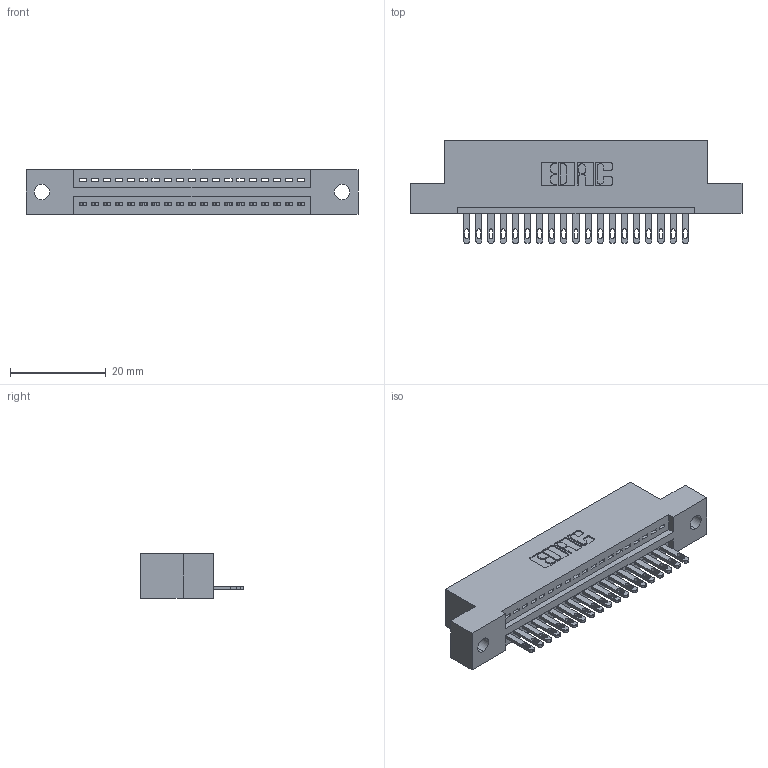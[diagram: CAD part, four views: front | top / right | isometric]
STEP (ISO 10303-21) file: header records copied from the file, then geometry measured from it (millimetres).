
FILE_DESCRIPTION (( 'STEP AP203' ), '1' );
FILE_NAME ('895-019-500-102.STEP', '2020-09-25T06:59:37', ( '' ), ( '' ), 'SwSTEP 2.0', 'SolidWorks 2020', '' );
FILE_SCHEMA (( 'CONFIG_CONTROL_DESIGN' ));
Length unit declared in the file: inch
Products named in the file (3): 345-292-001_345-293-100; 895-019-500-102; 845 Part_Flush Mounting Lugs - 0.128 Dia
Assembly tree (20 placements, depth 2):
  895-019-500-102
    845 Part_Flush Mounting Lugs - 0.128 Dia
    345-292-001_345-293-100  x19
Bounding box: 69.47 x 21.51 x 9.4 mm (x, y, z)
Volume: 6384.9 mm3; surface area: 7943.5 mm2
Topology: 20 solids, 20 shells, 1152 faces, 3533 edges, 2354 vertices
Faces by surface type: plane 726, cylinder 426
Entity records: 17329 total; most frequent: CARTESIAN_POINT 3009, ORIENTED_EDGE 2962, DIRECTION 2663, EDGE_CURVE 1481, LINE 1269, VECTOR 1269, VERTEX_POINT 986, AXIS2_PLACEMENT_3D 697
